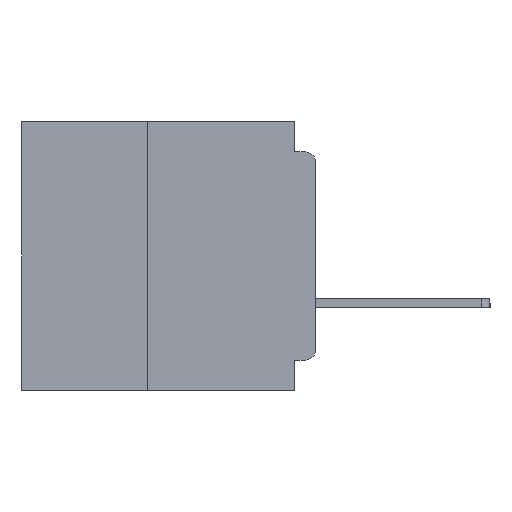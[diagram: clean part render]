
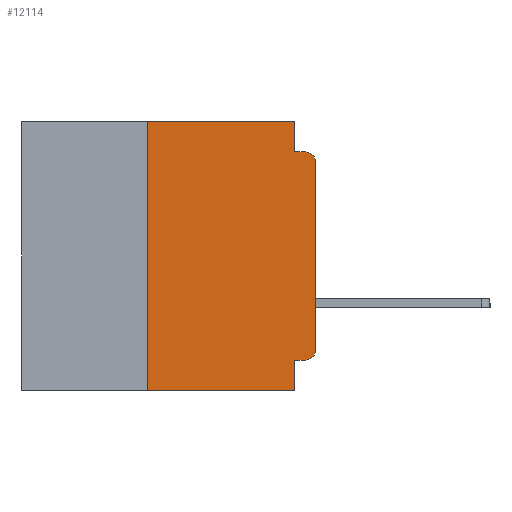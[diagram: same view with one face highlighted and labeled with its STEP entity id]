
A CAD part, left-side view. The second image highlights one B-rep face of the part: STEP entity #12114.
In plain terms, the highlighted planar face has unit normal (-1, 0, 0).
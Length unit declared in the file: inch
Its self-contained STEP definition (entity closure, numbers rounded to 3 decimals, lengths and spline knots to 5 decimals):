
#2393 = CARTESIAN_POINT ( 'NONE',  ( 0., 0.031, -0.4 ) ) ;
#4150 = VECTOR ( 'NONE', #31843, 39.37008 ) ;
#4344 = VERTEX_POINT ( 'NONE', #29059 ) ;
#5130 = LINE ( 'NONE', #35005, #4150 ) ;
#5185 = CARTESIAN_POINT ( 'NONE',  ( 0., 0., -0.06 ) ) ;
#5818 = CIRCLE ( 'NONE', #7690, 0.015 ) ;
#5936 = ORIENTED_EDGE ( 'NONE', *, *, #35753, .F. ) ;
#6142 = LINE ( 'NONE', #18143, #13622 ) ;
#7181 = VERTEX_POINT ( 'NONE', #14460 ) ;
#7690 = AXIS2_PLACEMENT_3D ( 'NONE', #17092, #39301, #20341 ) ;
#7951 = LINE ( 'NONE', #30958, #40785 ) ;
#8943 = ORIENTED_EDGE ( 'NONE', *, *, #16527, .T. ) ;
#9267 = CARTESIAN_POINT ( 'NONE',  ( 0., 0.25, -0.4 ) ) ;
#9272 = EDGE_CURVE ( 'NONE', #31762, #38404, #5818, .T. ) ;
#9353 = ORIENTED_EDGE ( 'NONE', *, *, #9272, .T. ) ;
#11049 = CARTESIAN_POINT ( 'NONE',  ( 0., 0.015, -0.34 ) ) ;
#11876 = DIRECTION ( 'NONE',  ( 0., 0., 1. ) ) ;
#12114 = ADVANCED_FACE ( 'NONE', ( #37967 ), #15334, .F. ) ;
#12138 = EDGE_LOOP ( 'NONE', ( #16804, #9353, #36662, #37065, #5936, #20584, #19811, #35157, #14692, #8943 ) ) ;
#12536 = AXIS2_PLACEMENT_3D ( 'NONE', #34366, #37565, #18546 ) ;
#13311 = CARTESIAN_POINT ( 'NONE',  ( 0., 0.015, -0.355 ) ) ;
#13622 = VECTOR ( 'NONE', #21404, 39.37008 ) ;
#13816 = VERTEX_POINT ( 'NONE', #20814 ) ;
#14322 = DIRECTION ( 'NONE',  ( 0., 0., -1. ) ) ;
#14460 = CARTESIAN_POINT ( 'NONE',  ( 0., 0.031, -0.045 ) ) ;
#14692 = ORIENTED_EDGE ( 'NONE', *, *, #34912, .F. ) ;
#15334 = PLANE ( 'NONE',  #12536 ) ;
#15376 = CARTESIAN_POINT ( 'NONE',  ( 0., 0.437, -0.4 ) ) ;
#16527 = EDGE_CURVE ( 'NONE', #33223, #4344, #23620, .T. ) ;
#16555 = VECTOR ( 'NONE', #36291, 39.37008 ) ;
#16804 = ORIENTED_EDGE ( 'NONE', *, *, #24063, .T. ) ;
#17092 = CARTESIAN_POINT ( 'NONE',  ( 0., 0.015, -0.06 ) ) ;
#17670 = LINE ( 'NONE', #30879, #24181 ) ;
#17782 = CARTESIAN_POINT ( 'NONE',  ( 0., 0.25, -0.4 ) ) ;
#17993 = EDGE_CURVE ( 'NONE', #31659, #32693, #34378, .T. ) ;
#18143 = CARTESIAN_POINT ( 'NONE',  ( 0., 0., -0.045 ) ) ;
#18546 = DIRECTION ( 'NONE',  ( 0., 0., -1. ) ) ;
#18607 = CARTESIAN_POINT ( 'NONE',  ( 0., 0.015, -0.045 ) ) ;
#19811 = ORIENTED_EDGE ( 'NONE', *, *, #35823, .T. ) ;
#20341 = DIRECTION ( 'NONE',  ( 0., 0., -1. ) ) ;
#20584 = ORIENTED_EDGE ( 'NONE', *, *, #17993, .F. ) ;
#20814 = CARTESIAN_POINT ( 'NONE',  ( 0., 0.031, -0.355 ) ) ;
#21404 = DIRECTION ( 'NONE',  ( 0., -1., 0. ) ) ;
#21628 = VERTEX_POINT ( 'NONE', #2393 ) ;
#21853 = VECTOR ( 'NONE', #24049, 39.37008 ) ;
#22000 = VECTOR ( 'NONE', #28176, 39.37008 ) ;
#22131 = AXIS2_PLACEMENT_3D ( 'NONE', #11049, #33387, #14322 ) ;
#23620 = CIRCLE ( 'NONE', #22131, 0.015 ) ;
#24049 = DIRECTION ( 'NONE',  ( 0., 0., -1. ) ) ;
#24063 = EDGE_CURVE ( 'NONE', #4344, #31762, #17670, .T. ) ;
#24181 = VECTOR ( 'NONE', #11876, 39.37008 ) ;
#25945 = VECTOR ( 'NONE', #40118, 39.37008 ) ;
#26948 = EDGE_CURVE ( 'NONE', #7181, #38404, #6142, .T. ) ;
#28176 = DIRECTION ( 'NONE',  ( 0., -1., 0. ) ) ;
#29059 = CARTESIAN_POINT ( 'NONE',  ( 0., 0., -0.34 ) ) ;
#29452 = CARTESIAN_POINT ( 'NONE',  ( 0., 0.031, 0. ) ) ;
#29905 = CARTESIAN_POINT ( 'NONE',  ( 0., 0., -0.355 ) ) ;
#30266 = CARTESIAN_POINT ( 'NONE',  ( 0., 0.031, 0. ) ) ;
#30621 = VERTEX_POINT ( 'NONE', #29452 ) ;
#30782 = EDGE_CURVE ( 'NONE', #30621, #7181, #38679, .T. ) ;
#30879 = CARTESIAN_POINT ( 'NONE',  ( 0., 0., 0. ) ) ;
#30958 = CARTESIAN_POINT ( 'NONE',  ( 0., 0.437, 0. ) ) ;
#31659 = VERTEX_POINT ( 'NONE', #9267 ) ;
#31762 = VERTEX_POINT ( 'NONE', #5185 ) ;
#31843 = DIRECTION ( 'NONE',  ( 0., 0., -1. ) ) ;
#32693 = VERTEX_POINT ( 'NONE', #35358 ) ;
#33223 = VERTEX_POINT ( 'NONE', #13311 ) ;
#33387 = DIRECTION ( 'NONE',  ( -1., 0., 0. ) ) ;
#33697 = EDGE_CURVE ( 'NONE', #13816, #21628, #5130, .T. ) ;
#34366 = CARTESIAN_POINT ( 'NONE',  ( 0., 0.437, 0. ) ) ;
#34378 = LINE ( 'NONE', #17782, #25945 ) ;
#34912 = EDGE_CURVE ( 'NONE', #33223, #13816, #40859, .T. ) ;
#35005 = CARTESIAN_POINT ( 'NONE',  ( 0., 0.031, -0.4 ) ) ;
#35157 = ORIENTED_EDGE ( 'NONE', *, *, #33697, .F. ) ;
#35358 = CARTESIAN_POINT ( 'NONE',  ( 0., 0.25, 0. ) ) ;
#35753 = EDGE_CURVE ( 'NONE', #32693, #30621, #7951, .T. ) ;
#35823 = EDGE_CURVE ( 'NONE', #31659, #21628, #38827, .T. ) ;
#36291 = DIRECTION ( 'NONE',  ( 0., 1., 0. ) ) ;
#36662 = ORIENTED_EDGE ( 'NONE', *, *, #26948, .F. ) ;
#37065 = ORIENTED_EDGE ( 'NONE', *, *, #30782, .F. ) ;
#37338 = DIRECTION ( 'NONE',  ( 0., -1., 0. ) ) ;
#37565 = DIRECTION ( 'NONE',  ( 1., 0., 0. ) ) ;
#37967 = FACE_OUTER_BOUND ( 'NONE', #12138, .T. ) ;
#38404 = VERTEX_POINT ( 'NONE', #18607 ) ;
#38679 = LINE ( 'NONE', #30266, #21853 ) ;
#38827 = LINE ( 'NONE', #15376, #22000 ) ;
#39301 = DIRECTION ( 'NONE',  ( -1., 0., 0. ) ) ;
#40118 = DIRECTION ( 'NONE',  ( 0., 0., 1. ) ) ;
#40785 = VECTOR ( 'NONE', #37338, 39.37008 ) ;
#40859 = LINE ( 'NONE', #29905, #16555 ) ;
